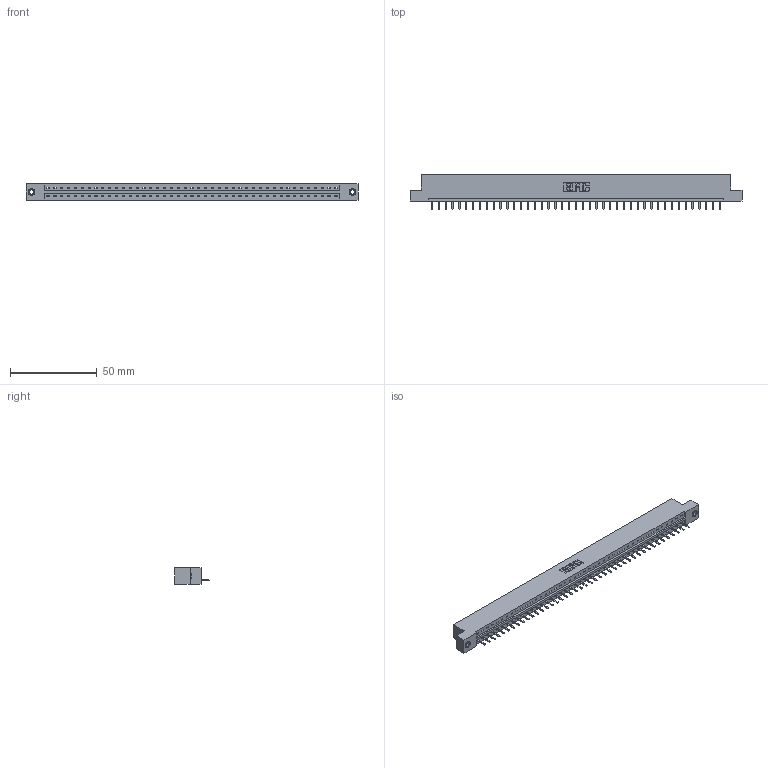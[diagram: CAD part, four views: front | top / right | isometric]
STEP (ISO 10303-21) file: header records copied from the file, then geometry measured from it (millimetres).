
FILE_DESCRIPTION (( 'STEP AP203' ), '1' );
FILE_NAME ('333-043-520-107.STEP', '2018-08-03T20:00:29', ( '' ), ( '' ), 'SwSTEP 2.0', 'SolidWorks 2016', '' );
FILE_SCHEMA (( 'CONFIG_CONTROL_DESIGN' ));
Length unit declared in the file: inch
Products named in the file (4): 333-043-520-107; 333 Part_Flush - .156 Dia - TI; 345-292-001_345-293-120; 345-250-001_345-250-005-103
Assembly tree (46 placements, depth 2):
  333-043-520-107
    333 Part_Flush - .156 Dia - TI
    345-292-001_345-293-120  x43
    345-250-001_345-250-005-103  x2
Bounding box: 191.92 x 20.02 x 9.4 mm (x, y, z)
Volume: 19184.2 mm3; surface area: 20367.2 mm2
Topology: 46 solids, 46 shells, 2840 faces, 8359 edges, 5450 vertices
Faces by surface type: plane 1994, cylinder 830, cone 12, torus 4
Entity records: 27458 total; most frequent: CARTESIAN_POINT 4730, ORIENTED_EDGE 4690, DIRECTION 4009, EDGE_CURVE 2345, VECTOR 2193, LINE 2193, VERTEX_POINT 1556, AXIS2_PLACEMENT_3D 908
